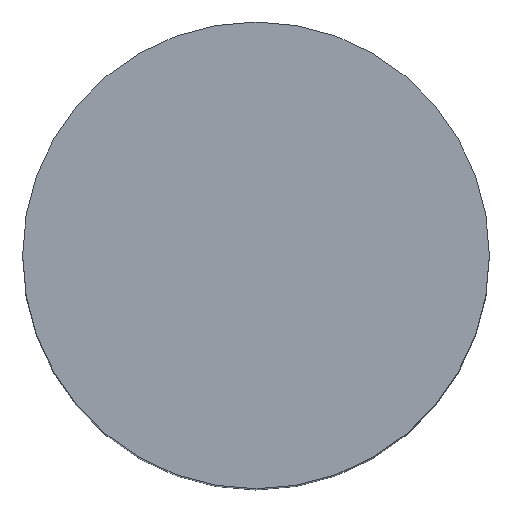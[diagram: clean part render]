
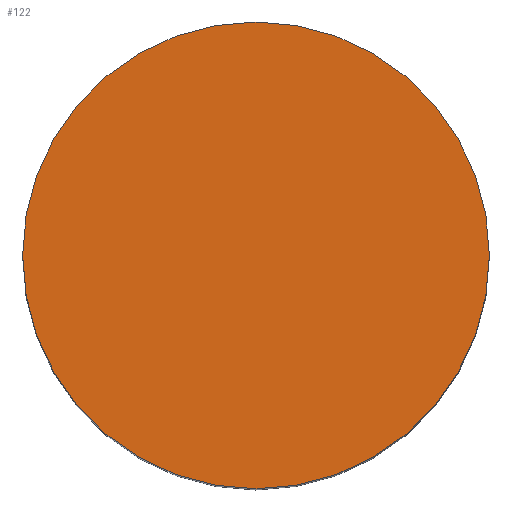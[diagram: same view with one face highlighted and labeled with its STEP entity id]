
A CAD part, top view. The second image highlights one B-rep face of the part: STEP entity #122.
In plain terms, the highlighted planar face has unit normal (0, 0, 1).
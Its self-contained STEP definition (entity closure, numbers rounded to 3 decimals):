
#9 = CARTESIAN_POINT ( 'NONE',  ( -2.5, 0., 3.75 ) ) ;
#13 = CARTESIAN_POINT ( 'NONE',  ( 0., 0., 3.75 ) ) ;
#17 = DIRECTION ( 'NONE',  ( 1., 0., 0. ) ) ;
#24 = DIRECTION ( 'NONE',  ( 1., 0., 0. ) ) ;
#28 = DIRECTION ( 'NONE',  ( 0., 0., 1. ) ) ;
#36 = EDGE_CURVE ( 'NONE', #72, #102, #67, .T. ) ;
#48 = EDGE_CURVE ( 'NONE', #102, #72, #68, .T. ) ;
#53 = DIRECTION ( 'NONE',  ( 0., 0., 1. ) ) ;
#58 = AXIS2_PLACEMENT_3D ( 'NONE', #74, #28, #17 ) ;
#59 = EDGE_LOOP ( 'NONE', ( #121, #60 ) ) ;
#60 = ORIENTED_EDGE ( 'NONE', *, *, #48, .T. ) ;
#64 = PLANE ( 'NONE',  #58 ) ;
#67 = CIRCLE ( 'NONE', #126, 2.5 ) ;
#68 = CIRCLE ( 'NONE', #119, 2.5 ) ;
#70 = FACE_OUTER_BOUND ( 'NONE', #59, .T. ) ;
#72 = VERTEX_POINT ( 'NONE', #9 ) ;
#74 = CARTESIAN_POINT ( 'NONE',  ( 0., 0., 3.75 ) ) ;
#77 = CARTESIAN_POINT ( 'NONE',  ( 2.5, 0., 3.75 ) ) ;
#95 = DIRECTION ( 'NONE',  ( 0., 0., 1. ) ) ;
#102 = VERTEX_POINT ( 'NONE', #77 ) ;
#115 = CARTESIAN_POINT ( 'NONE',  ( 0., 0., 3.75 ) ) ;
#119 = AXIS2_PLACEMENT_3D ( 'NONE', #115, #53, #125 ) ;
#121 = ORIENTED_EDGE ( 'NONE', *, *, #36, .T. ) ;
#122 = ADVANCED_FACE ( 'NONE', ( #70 ), #64, .T. ) ;
#125 = DIRECTION ( 'NONE',  ( 1., 0., 0. ) ) ;
#126 = AXIS2_PLACEMENT_3D ( 'NONE', #13, #95, #24 ) ;
